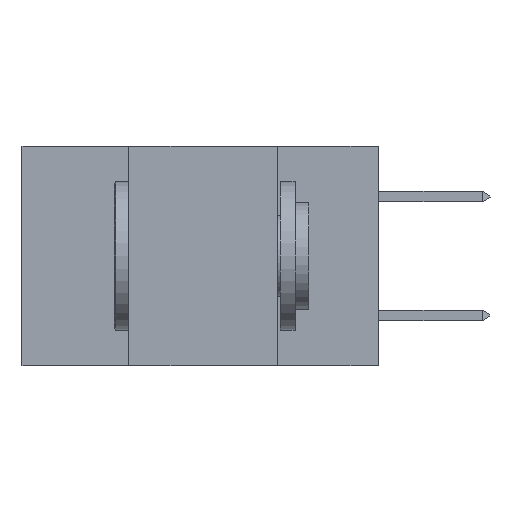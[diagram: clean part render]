
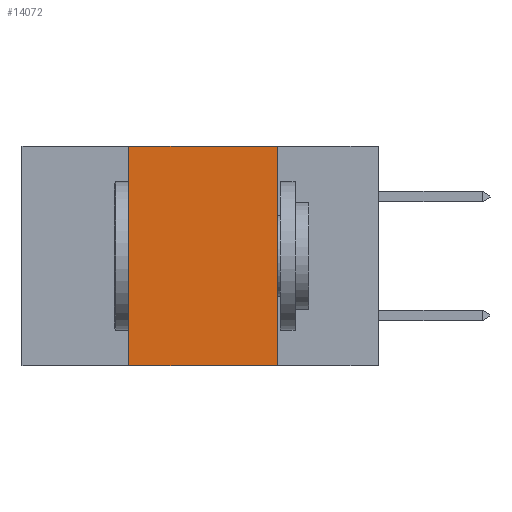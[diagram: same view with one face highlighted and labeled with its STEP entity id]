
A CAD part, left-side view. The second image highlights one B-rep face of the part: STEP entity #14072.
In plain terms, the highlighted planar face has unit normal (-1, 0, 0).
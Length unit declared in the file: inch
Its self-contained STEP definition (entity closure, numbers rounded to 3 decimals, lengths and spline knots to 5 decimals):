
#435 = CARTESIAN_POINT ( 'NONE',  ( 0., 0.6, 0. ) ) ;
#535 = VERTEX_POINT ( 'NONE', #6440 ) ;
#1956 = VERTEX_POINT ( 'NONE', #16819 ) ;
#2499 = DIRECTION ( 'NONE',  ( 0., 0., -1. ) ) ;
#2997 = EDGE_CURVE ( 'NONE', #15767, #535, #6742, .T. ) ;
#4432 = EDGE_LOOP ( 'NONE', ( #10236, #9758, #10697, #11351 ) ) ;
#4620 = EDGE_CURVE ( 'NONE', #535, #9847, #15712, .T. ) ;
#4672 = EDGE_CURVE ( 'NONE', #1956, #15767, #11430, .T. ) ;
#4705 = EDGE_CURVE ( 'NONE', #1956, #9847, #14875, .T. ) ;
#5478 = CARTESIAN_POINT ( 'NONE',  ( 0., 0.17, 0. ) ) ;
#5998 = AXIS2_PLACEMENT_3D ( 'NONE', #435, #16973, #8118 ) ;
#6440 = CARTESIAN_POINT ( 'NONE',  ( 0., 0.17, 0. ) ) ;
#6627 = PLANE ( 'NONE',  #5998 ) ;
#6742 = LINE ( 'NONE', #18259, #10285 ) ;
#6922 = DIRECTION ( 'NONE',  ( 0., -1., 0. ) ) ;
#7343 = VECTOR ( 'NONE', #2499, 39.37008 ) ;
#8118 = DIRECTION ( 'NONE',  ( 0., 0., -1. ) ) ;
#8698 = CARTESIAN_POINT ( 'NONE',  ( 0., 0.6, -0.37 ) ) ;
#9758 = ORIENTED_EDGE ( 'NONE', *, *, #2997, .F. ) ;
#9847 = VERTEX_POINT ( 'NONE', #12310 ) ;
#9987 = CARTESIAN_POINT ( 'NONE',  ( 0., 0.42, 0. ) ) ;
#10236 = ORIENTED_EDGE ( 'NONE', *, *, #4620, .F. ) ;
#10285 = VECTOR ( 'NONE', #13268, 39.37008 ) ;
#10526 = VECTOR ( 'NONE', #6922, 39.37008 ) ;
#10697 = ORIENTED_EDGE ( 'NONE', *, *, #4672, .F. ) ;
#11063 = FACE_OUTER_BOUND ( 'NONE', #4432, .T. ) ;
#11351 = ORIENTED_EDGE ( 'NONE', *, *, #4705, .T. ) ;
#11430 = LINE ( 'NONE', #13802, #18678 ) ;
#12310 = CARTESIAN_POINT ( 'NONE',  ( 0., 0.17, -0.37 ) ) ;
#12839 = DIRECTION ( 'NONE',  ( 0., 0., 1. ) ) ;
#13268 = DIRECTION ( 'NONE',  ( 0., -1., 0. ) ) ;
#13802 = CARTESIAN_POINT ( 'NONE',  ( 0., 0.42, 0. ) ) ;
#14072 = ADVANCED_FACE ( 'NONE', ( #11063 ), #6627, .F. ) ;
#14875 = LINE ( 'NONE', #8698, #10526 ) ;
#15712 = LINE ( 'NONE', #5478, #7343 ) ;
#15767 = VERTEX_POINT ( 'NONE', #9987 ) ;
#16819 = CARTESIAN_POINT ( 'NONE',  ( 0., 0.42, -0.37 ) ) ;
#16973 = DIRECTION ( 'NONE',  ( 1., 0., 0. ) ) ;
#18259 = CARTESIAN_POINT ( 'NONE',  ( 0., 0.6, 0. ) ) ;
#18678 = VECTOR ( 'NONE', #12839, 39.37008 ) ;
